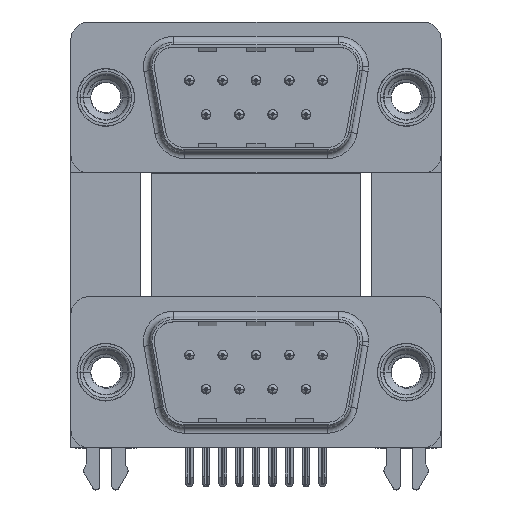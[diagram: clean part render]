
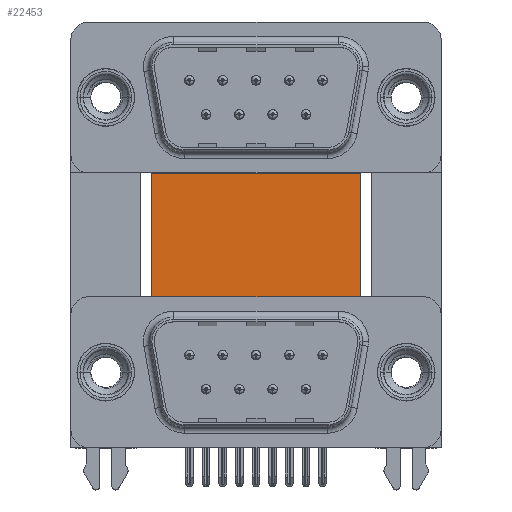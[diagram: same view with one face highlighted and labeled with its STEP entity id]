
A CAD part, top view. The second image highlights one B-rep face of the part: STEP entity #22453.
In plain terms, the highlighted planar face has unit normal (0, 0, 1).
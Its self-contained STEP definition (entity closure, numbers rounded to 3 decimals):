
#14 = CARTESIAN_POINT ( 'NONE',  ( 2.9, -3.735, -12. ) ) ;
#1036 = DIRECTION ( 'NONE',  ( 0., -1., 0. ) ) ;
#1676 = CARTESIAN_POINT ( 'NONE',  ( 22.59, -4.635, -12. ) ) ;
#1897 = DIRECTION ( 'NONE',  ( 0., -1., 0. ) ) ;
#1934 = VECTOR ( 'NONE', #10634, 1000. ) ;
#2131 = VERTEX_POINT ( 'NONE', #11656 ) ;
#2334 = CARTESIAN_POINT ( 'NONE',  ( 2.4, -4.635, -12. ) ) ;
#2336 = ORIENTED_EDGE ( 'NONE', *, *, #8535, .T. ) ;
#2364 = CARTESIAN_POINT ( 'NONE',  ( 3.79, 16.585, -12. ) ) ;
#2870 = CARTESIAN_POINT ( 'NONE',  ( 22.09, -4.635, -12. ) ) ;
#3352 = VERTEX_POINT ( 'NONE', #1676 ) ;
#3521 = CARTESIAN_POINT ( 'NONE',  ( 22.09, -4.635, -12. ) ) ;
#4023 = EDGE_CURVE ( 'NONE', #4915, #3352, #7457, .T. ) ;
#4355 = EDGE_CURVE ( 'NONE', #13918, #9394, #11431, .T. ) ;
#4648 = EDGE_LOOP ( 'NONE', ( #8312, #5507, #13480, #25353, #13438, #18773, #2336, #8862, #15327, #23385 ) ) ;
#4858 = VECTOR ( 'NONE', #6357, 1000. ) ;
#4915 = VERTEX_POINT ( 'NONE', #3521 ) ;
#5507 = ORIENTED_EDGE ( 'NONE', *, *, #15532, .T. ) ;
#5597 = EDGE_CURVE ( 'NONE', #7386, #2131, #15548, .T. ) ;
#5862 = VERTEX_POINT ( 'NONE', #12081 ) ;
#6357 = DIRECTION ( 'NONE',  ( -0.336, -0.942, 0. ) ) ;
#6383 = PLANE ( 'NONE',  #9878 ) ;
#6607 = EDGE_CURVE ( 'NONE', #2131, #19969, #11551, .T. ) ;
#7190 = CARTESIAN_POINT ( 'NONE',  ( 3.79, 16.585, -12. ) ) ;
#7386 = VERTEX_POINT ( 'NONE', #21439 ) ;
#7457 = LINE ( 'NONE', #2870, #21057 ) ;
#8312 = ORIENTED_EDGE ( 'NONE', *, *, #4355, .T. ) ;
#8436 = EDGE_CURVE ( 'NONE', #14015, #5862, #15705, .T. ) ;
#8535 = EDGE_CURVE ( 'NONE', #14015, #7386, #20998, .T. ) ;
#8776 = LINE ( 'NONE', #14, #27754 ) ;
#8862 = ORIENTED_EDGE ( 'NONE', *, *, #5597, .T. ) ;
#9394 = VERTEX_POINT ( 'NONE', #19396 ) ;
#9594 = DIRECTION ( 'NONE',  ( 1., 0., 0. ) ) ;
#9878 = AXIS2_PLACEMENT_3D ( 'NONE', #2364, #22200, #26375 ) ;
#10056 = CARTESIAN_POINT ( 'NONE',  ( 3.79, 16.585, -12. ) ) ;
#10451 = VERTEX_POINT ( 'NONE', #12338 ) ;
#10634 = DIRECTION ( 'NONE',  ( 0., -1., 0. ) ) ;
#11235 = DIRECTION ( 'NONE',  ( 1., 0., 0. ) ) ;
#11431 = LINE ( 'NONE', #26708, #14181 ) ;
#11551 = LINE ( 'NONE', #13581, #18139 ) ;
#11656 = CARTESIAN_POINT ( 'NONE',  ( 2.4, -4.635, -12. ) ) ;
#12081 = CARTESIAN_POINT ( 'NONE',  ( 21.2, 16.585, -12. ) ) ;
#12338 = CARTESIAN_POINT ( 'NONE',  ( 21.2, -0.735, -12. ) ) ;
#13252 = CARTESIAN_POINT ( 'NONE',  ( 3.79, 16.585, -12. ) ) ;
#13387 = CARTESIAN_POINT ( 'NONE',  ( 2.9, -3.735, -12. ) ) ;
#13438 = ORIENTED_EDGE ( 'NONE', *, *, #24685, .F. ) ;
#13480 = ORIENTED_EDGE ( 'NONE', *, *, #4023, .T. ) ;
#13581 = CARTESIAN_POINT ( 'NONE',  ( 2.9, -4.635, -12. ) ) ;
#13918 = VERTEX_POINT ( 'NONE', #13387 ) ;
#14015 = VERTEX_POINT ( 'NONE', #7190 ) ;
#14181 = VECTOR ( 'NONE', #20370, 1000. ) ;
#14968 = LINE ( 'NONE', #24025, #1934 ) ;
#14979 = DIRECTION ( 'NONE',  ( 0., 1., 0. ) ) ;
#15327 = ORIENTED_EDGE ( 'NONE', *, *, #6607, .T. ) ;
#15532 = EDGE_CURVE ( 'NONE', #9394, #4915, #23307, .T. ) ;
#15548 = LINE ( 'NONE', #2334, #4858 ) ;
#15705 = LINE ( 'NONE', #13252, #27067 ) ;
#17317 = FACE_OUTER_BOUND ( 'NONE', #4648, .T. ) ;
#18139 = VECTOR ( 'NONE', #26809, 1000. ) ;
#18773 = ORIENTED_EDGE ( 'NONE', *, *, #8436, .F. ) ;
#19377 = CARTESIAN_POINT ( 'NONE',  ( 22.59, -4.635, -12. ) ) ;
#19396 = CARTESIAN_POINT ( 'NONE',  ( 22.09, -3.735, -12. ) ) ;
#19969 = VERTEX_POINT ( 'NONE', #20585 ) ;
#20370 = DIRECTION ( 'NONE',  ( 1., 0., 0. ) ) ;
#20585 = CARTESIAN_POINT ( 'NONE',  ( 2.9, -4.635, -12. ) ) ;
#20998 = LINE ( 'NONE', #10056, #23839 ) ;
#21057 = VECTOR ( 'NONE', #9594, 1000. ) ;
#21439 = CARTESIAN_POINT ( 'NONE',  ( 3.79, -0.735, -12. ) ) ;
#21498 = EDGE_CURVE ( 'NONE', #19969, #13918, #8776, .T. ) ;
#22200 = DIRECTION ( 'NONE',  ( 0., 0., -1. ) ) ;
#22453 = ADVANCED_FACE ( 'NONE', ( #17317 ), #6383, .F. ) ;
#23307 = LINE ( 'NONE', #25897, #26243 ) ;
#23385 = ORIENTED_EDGE ( 'NONE', *, *, #21498, .T. ) ;
#23446 = VECTOR ( 'NONE', #26118, 1000. ) ;
#23734 = EDGE_CURVE ( 'NONE', #3352, #10451, #28281, .T. ) ;
#23839 = VECTOR ( 'NONE', #1036, 1000. ) ;
#24025 = CARTESIAN_POINT ( 'NONE',  ( 21.2, 16.585, -12. ) ) ;
#24685 = EDGE_CURVE ( 'NONE', #5862, #10451, #14968, .T. ) ;
#25353 = ORIENTED_EDGE ( 'NONE', *, *, #23734, .T. ) ;
#25897 = CARTESIAN_POINT ( 'NONE',  ( 22.09, -3.735, -12. ) ) ;
#26118 = DIRECTION ( 'NONE',  ( -0.336, 0.942, 0. ) ) ;
#26243 = VECTOR ( 'NONE', #1897, 1000. ) ;
#26375 = DIRECTION ( 'NONE',  ( -1., 0., 0. ) ) ;
#26708 = CARTESIAN_POINT ( 'NONE',  ( 3.79, -3.735, -12. ) ) ;
#26809 = DIRECTION ( 'NONE',  ( 1., 0., 0. ) ) ;
#27067 = VECTOR ( 'NONE', #11235, 1000. ) ;
#27754 = VECTOR ( 'NONE', #14979, 1000. ) ;
#28281 = LINE ( 'NONE', #19377, #23446 ) ;
